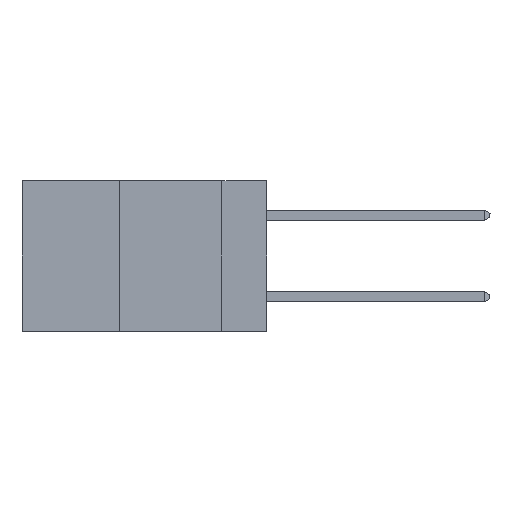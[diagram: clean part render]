
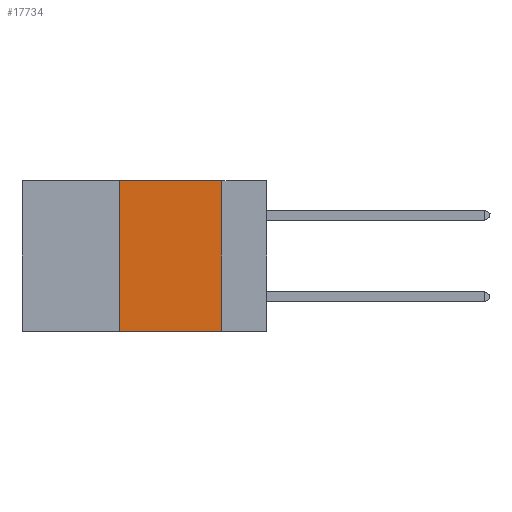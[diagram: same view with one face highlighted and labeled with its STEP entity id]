
A CAD part, left-side view. The second image highlights one B-rep face of the part: STEP entity #17734.
In plain terms, the highlighted planar face has unit normal (-1, 0, 0).
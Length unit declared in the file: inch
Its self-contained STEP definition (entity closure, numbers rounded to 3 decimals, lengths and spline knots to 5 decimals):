
#642 = EDGE_LOOP ( 'NONE', ( #10989, #23727, #13789, #8150 ) ) ;
#711 = LINE ( 'NONE', #4942, #15789 ) ;
#1477 = DIRECTION ( 'NONE',  ( 0., -1., 0. ) ) ;
#1572 = CARTESIAN_POINT ( 'NONE',  ( 0., 0.11, 0. ) ) ;
#1849 = CARTESIAN_POINT ( 'NONE',  ( 0., 0.6, 0. ) ) ;
#2834 = CARTESIAN_POINT ( 'NONE',  ( 0., 0.36, -0.37 ) ) ;
#3170 = CARTESIAN_POINT ( 'NONE',  ( 0., 0.11, 0. ) ) ;
#3400 = CARTESIAN_POINT ( 'NONE',  ( 0., 0.6, 0. ) ) ;
#4942 = CARTESIAN_POINT ( 'NONE',  ( 0., 0.36, 0. ) ) ;
#4965 = AXIS2_PLACEMENT_3D ( 'NONE', #3400, #11887, #22542 ) ;
#5206 = CARTESIAN_POINT ( 'NONE',  ( 0., 0.11, -0.37 ) ) ;
#5312 = VECTOR ( 'NONE', #1477, 39.37008 ) ;
#5539 = DIRECTION ( 'NONE',  ( 0., 0., -1. ) ) ;
#6805 = EDGE_CURVE ( 'NONE', #22287, #8198, #9525, .T. ) ;
#7500 = VERTEX_POINT ( 'NONE', #26631 ) ;
#8150 = ORIENTED_EDGE ( 'NONE', *, *, #6805, .T. ) ;
#8198 = VERTEX_POINT ( 'NONE', #5206 ) ;
#8395 = DIRECTION ( 'NONE',  ( 0., -1., 0. ) ) ;
#9525 = LINE ( 'NONE', #22259, #5312 ) ;
#10989 = ORIENTED_EDGE ( 'NONE', *, *, #15182, .F. ) ;
#11887 = DIRECTION ( 'NONE',  ( 1., 0., 0. ) ) ;
#13789 = ORIENTED_EDGE ( 'NONE', *, *, #14775, .F. ) ;
#14775 = EDGE_CURVE ( 'NONE', #22287, #7500, #711, .T. ) ;
#15152 = VECTOR ( 'NONE', #8395, 39.37008 ) ;
#15182 = EDGE_CURVE ( 'NONE', #15945, #8198, #17976, .T. ) ;
#15789 = VECTOR ( 'NONE', #25906, 39.37008 ) ;
#15945 = VERTEX_POINT ( 'NONE', #3170 ) ;
#16478 = LINE ( 'NONE', #1849, #15152 ) ;
#17734 = ADVANCED_FACE ( 'NONE', ( #22148 ), #17884, .F. ) ;
#17884 = PLANE ( 'NONE',  #4965 ) ;
#17976 = LINE ( 'NONE', #1572, #26326 ) ;
#22148 = FACE_OUTER_BOUND ( 'NONE', #642, .T. ) ;
#22259 = CARTESIAN_POINT ( 'NONE',  ( 0., 0.6, -0.37 ) ) ;
#22287 = VERTEX_POINT ( 'NONE', #2834 ) ;
#22542 = DIRECTION ( 'NONE',  ( 0., 0., -1. ) ) ;
#22623 = EDGE_CURVE ( 'NONE', #7500, #15945, #16478, .T. ) ;
#23727 = ORIENTED_EDGE ( 'NONE', *, *, #22623, .F. ) ;
#25906 = DIRECTION ( 'NONE',  ( 0., 0., 1. ) ) ;
#26326 = VECTOR ( 'NONE', #5539, 39.37008 ) ;
#26631 = CARTESIAN_POINT ( 'NONE',  ( 0., 0.36, 0. ) ) ;
